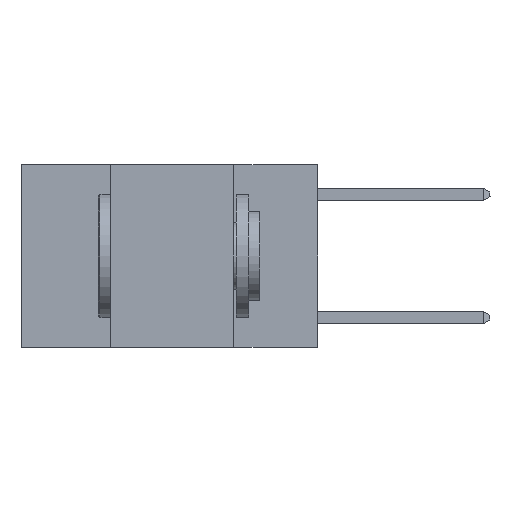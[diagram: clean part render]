
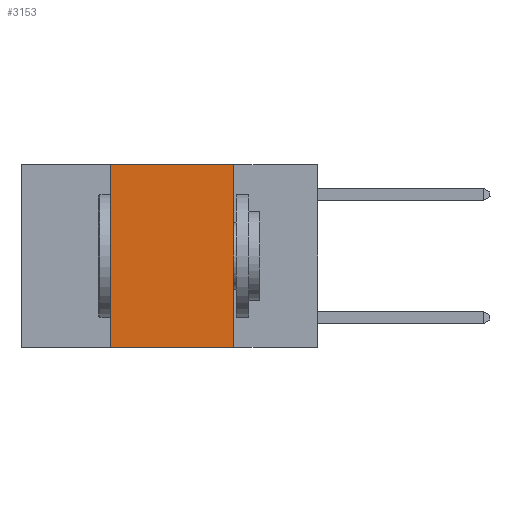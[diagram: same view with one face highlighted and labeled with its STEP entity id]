
A CAD part, left-side view. The second image highlights one B-rep face of the part: STEP entity #3153.
In plain terms, the highlighted planar face has unit normal (-1, 0, 0).
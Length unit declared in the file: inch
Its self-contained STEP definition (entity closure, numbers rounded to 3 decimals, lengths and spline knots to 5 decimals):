
#327 = VECTOR ( 'NONE', #9527, 39.37008 ) ;
#338 = LINE ( 'NONE', #1044, #10351 ) ;
#599 = AXIS2_PLACEMENT_3D ( 'NONE', #9346, #3578, #10215 ) ;
#908 = ORIENTED_EDGE ( 'NONE', *, *, #8556, .F. ) ;
#1044 = CARTESIAN_POINT ( 'NONE',  ( 0., 0.42, 0. ) ) ;
#1283 = EDGE_LOOP ( 'NONE', ( #3693, #908, #9144, #5477 ) ) ;
#1397 = LINE ( 'NONE', #6939, #6556 ) ;
#1887 = VERTEX_POINT ( 'NONE', #10993 ) ;
#1898 = LINE ( 'NONE', #8352, #9412 ) ;
#1977 = VERTEX_POINT ( 'NONE', #3205 ) ;
#3153 = ADVANCED_FACE ( 'NONE', ( #6285 ), #5629, .F. ) ;
#3205 = CARTESIAN_POINT ( 'NONE',  ( 0., 0.17, 0. ) ) ;
#3578 = DIRECTION ( 'NONE',  ( 1., 0., 0. ) ) ;
#3693 = ORIENTED_EDGE ( 'NONE', *, *, #8634, .F. ) ;
#5477 = ORIENTED_EDGE ( 'NONE', *, *, #8472, .T. ) ;
#5629 = PLANE ( 'NONE',  #599 ) ;
#6091 = VERTEX_POINT ( 'NONE', #11550 ) ;
#6285 = FACE_OUTER_BOUND ( 'NONE', #1283, .T. ) ;
#6556 = VECTOR ( 'NONE', #7862, 39.37008 ) ;
#6939 = CARTESIAN_POINT ( 'NONE',  ( 0., 0.17, 0. ) ) ;
#6963 = CARTESIAN_POINT ( 'NONE',  ( 0., 0.42, 0. ) ) ;
#7862 = DIRECTION ( 'NONE',  ( 0., 0., -1. ) ) ;
#8270 = EDGE_CURVE ( 'NONE', #1887, #10722, #338, .T. ) ;
#8300 = LINE ( 'NONE', #8671, #327 ) ;
#8352 = CARTESIAN_POINT ( 'NONE',  ( 0., 0.6, -0.37 ) ) ;
#8472 = EDGE_CURVE ( 'NONE', #1887, #6091, #1898, .T. ) ;
#8556 = EDGE_CURVE ( 'NONE', #10722, #1977, #8300, .T. ) ;
#8634 = EDGE_CURVE ( 'NONE', #1977, #6091, #1397, .T. ) ;
#8671 = CARTESIAN_POINT ( 'NONE',  ( 0., 0.6, 0. ) ) ;
#9144 = ORIENTED_EDGE ( 'NONE', *, *, #8270, .F. ) ;
#9346 = CARTESIAN_POINT ( 'NONE',  ( 0., 0.6, 0. ) ) ;
#9412 = VECTOR ( 'NONE', #10958, 39.37008 ) ;
#9527 = DIRECTION ( 'NONE',  ( 0., -1., 0. ) ) ;
#9860 = DIRECTION ( 'NONE',  ( 0., 0., 1. ) ) ;
#10215 = DIRECTION ( 'NONE',  ( 0., 0., -1. ) ) ;
#10351 = VECTOR ( 'NONE', #9860, 39.37008 ) ;
#10722 = VERTEX_POINT ( 'NONE', #6963 ) ;
#10958 = DIRECTION ( 'NONE',  ( 0., -1., 0. ) ) ;
#10993 = CARTESIAN_POINT ( 'NONE',  ( 0., 0.42, -0.37 ) ) ;
#11550 = CARTESIAN_POINT ( 'NONE',  ( 0., 0.17, -0.37 ) ) ;
